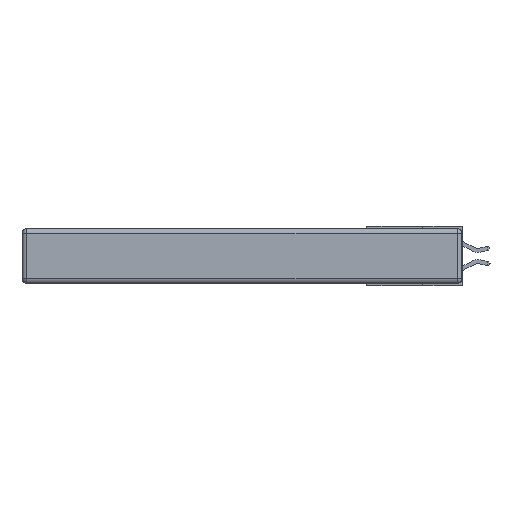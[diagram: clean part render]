
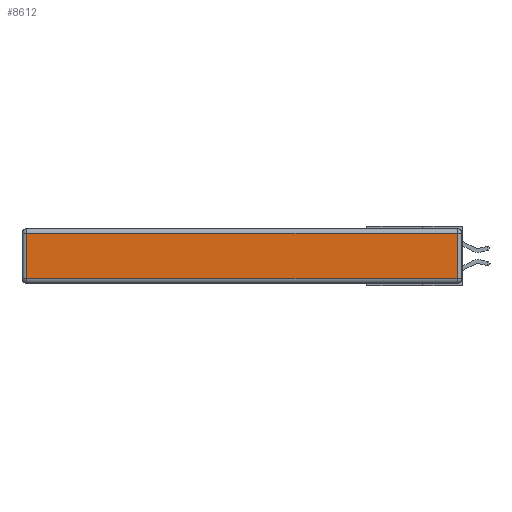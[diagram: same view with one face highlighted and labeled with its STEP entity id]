
A CAD part, left-side view. The second image highlights one B-rep face of the part: STEP entity #8612.
In plain terms, the highlighted planar face has unit normal (-1, 0, 0).
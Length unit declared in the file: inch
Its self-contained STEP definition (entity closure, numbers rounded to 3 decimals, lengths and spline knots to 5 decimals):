
#42 = ORIENTED_EDGE ( 'NONE', *, *, #4093, .T. ) ;
#157 = VECTOR ( 'NONE', #10028, 39.37008 ) ;
#369 = CARTESIAN_POINT ( 'NONE',  ( 0., 2.72, -0.03 ) ) ;
#919 = CARTESIAN_POINT ( 'NONE',  ( 0., 0.03, -0.343 ) ) ;
#1563 = EDGE_CURVE ( 'NONE', #10077, #11274, #5976, .T. ) ;
#1755 = PLANE ( 'NONE',  #11766 ) ;
#2396 = CARTESIAN_POINT ( 'NONE',  ( 0., 0.03, -0.313 ) ) ;
#3635 = EDGE_CURVE ( 'NONE', #11274, #19394, #13162, .T. ) ;
#4093 = EDGE_CURVE ( 'NONE', #19394, #4359, #14534, .T. ) ;
#4359 = VERTEX_POINT ( 'NONE', #2396 ) ;
#4568 = CARTESIAN_POINT ( 'NONE',  ( 0., 2.75, -0.03 ) ) ;
#4699 = DIRECTION ( 'NONE',  ( 0., 1., 0. ) ) ;
#5958 = DIRECTION ( 'NONE',  ( 0., 0., -1. ) ) ;
#5976 = LINE ( 'NONE', #4568, #13212 ) ;
#7085 = ORIENTED_EDGE ( 'NONE', *, *, #1563, .T. ) ;
#8612 = ADVANCED_FACE ( 'NONE', ( #13662 ), #1755, .T. ) ;
#9223 = CARTESIAN_POINT ( 'NONE',  ( 0., 0., -0.343 ) ) ;
#10028 = DIRECTION ( 'NONE',  ( 0., 0., 1. ) ) ;
#10077 = VERTEX_POINT ( 'NONE', #16718 ) ;
#10630 = VECTOR ( 'NONE', #5958, 39.37008 ) ;
#10737 = LINE ( 'NONE', #919, #157 ) ;
#11015 = EDGE_CURVE ( 'NONE', #4359, #10077, #10737, .T. ) ;
#11098 = EDGE_LOOP ( 'NONE', ( #42, #14408, #7085, #16402 ) ) ;
#11274 = VERTEX_POINT ( 'NONE', #369 ) ;
#11766 = AXIS2_PLACEMENT_3D ( 'NONE', #9223, #14938, #12005 ) ;
#12005 = DIRECTION ( 'NONE',  ( 0., 0., 1. ) ) ;
#13162 = LINE ( 'NONE', #14892, #10630 ) ;
#13212 = VECTOR ( 'NONE', #4699, 39.37008 ) ;
#13662 = FACE_OUTER_BOUND ( 'NONE', #11098, .T. ) ;
#14408 = ORIENTED_EDGE ( 'NONE', *, *, #11015, .T. ) ;
#14534 = LINE ( 'NONE', #17790, #18541 ) ;
#14892 = CARTESIAN_POINT ( 'NONE',  ( 0., 2.72, -0.343 ) ) ;
#14938 = DIRECTION ( 'NONE',  ( -1., 0., 0. ) ) ;
#16402 = ORIENTED_EDGE ( 'NONE', *, *, #3635, .T. ) ;
#16718 = CARTESIAN_POINT ( 'NONE',  ( 0., 0.03, -0.03 ) ) ;
#17790 = CARTESIAN_POINT ( 'NONE',  ( 0., 0., -0.313 ) ) ;
#17865 = DIRECTION ( 'NONE',  ( 0., -1., 0. ) ) ;
#18541 = VECTOR ( 'NONE', #17865, 39.37008 ) ;
#19247 = CARTESIAN_POINT ( 'NONE',  ( 0., 2.72, -0.313 ) ) ;
#19394 = VERTEX_POINT ( 'NONE', #19247 ) ;
